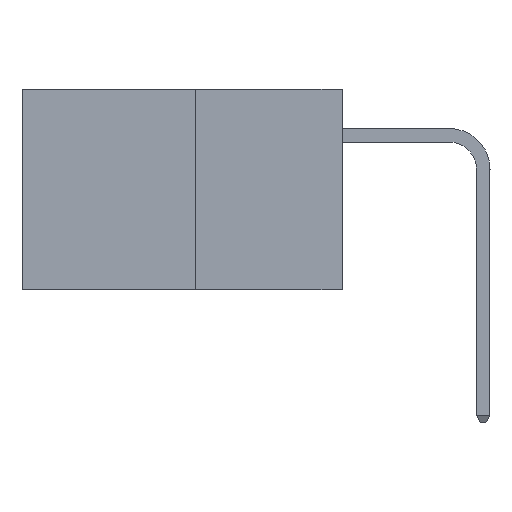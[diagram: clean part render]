
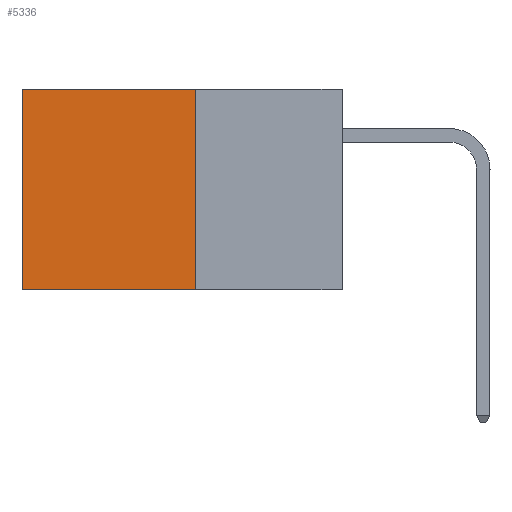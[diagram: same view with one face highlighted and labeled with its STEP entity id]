
A CAD part, left-side view. The second image highlights one B-rep face of the part: STEP entity #5336.
In plain terms, the highlighted planar face has unit normal (-1, 0, 0).
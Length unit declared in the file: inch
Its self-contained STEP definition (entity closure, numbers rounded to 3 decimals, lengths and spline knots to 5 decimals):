
#432 = EDGE_CURVE ( 'NONE', #10959, #10117, #7024, .T. ) ;
#1221 = ORIENTED_EDGE ( 'NONE', *, *, #6345, .F. ) ;
#1594 = ORIENTED_EDGE ( 'NONE', *, *, #6650, .F. ) ;
#2426 = FACE_OUTER_BOUND ( 'NONE', #8781, .T. ) ;
#2506 = CARTESIAN_POINT ( 'NONE',  ( 0.277, 0.27, -0.37 ) ) ;
#2788 = DIRECTION ( 'NONE',  ( 1., 0., 0. ) ) ;
#3275 = DIRECTION ( 'NONE',  ( 0., 0., -1. ) ) ;
#3583 = VECTOR ( 'NONE', #8710, 39.37008 ) ;
#3636 = EDGE_CURVE ( 'NONE', #10117, #7857, #12831, .T. ) ;
#4888 = VECTOR ( 'NONE', #12322, 39.37008 ) ;
#5064 = CARTESIAN_POINT ( 'NONE',  ( 0.277, 0.27, 0. ) ) ;
#5336 = ADVANCED_FACE ( 'NONE', ( #2426 ), #11012, .F. ) ;
#6202 = CARTESIAN_POINT ( 'NONE',  ( 0.277, 0.27, -0.37 ) ) ;
#6314 = LINE ( 'NONE', #2506, #3583 ) ;
#6345 = EDGE_CURVE ( 'NONE', #10959, #6708, #6314, .T. ) ;
#6650 = EDGE_CURVE ( 'NONE', #6708, #7857, #10659, .T. ) ;
#6708 = VERTEX_POINT ( 'NONE', #6202 ) ;
#6890 = CARTESIAN_POINT ( 'NONE',  ( 0.277, 0.59, 0. ) ) ;
#7024 = LINE ( 'NONE', #5064, #12454 ) ;
#7400 = VECTOR ( 'NONE', #3275, 39.37008 ) ;
#7857 = VERTEX_POINT ( 'NONE', #8082 ) ;
#8082 = CARTESIAN_POINT ( 'NONE',  ( 0.277, 0.59, -0.37 ) ) ;
#8710 = DIRECTION ( 'NONE',  ( 0., 0., -1. ) ) ;
#8769 = ORIENTED_EDGE ( 'NONE', *, *, #432, .T. ) ;
#8781 = EDGE_LOOP ( 'NONE', ( #10660, #1594, #1221, #8769 ) ) ;
#8976 = AXIS2_PLACEMENT_3D ( 'NONE', #8977, #2788, #10025 ) ;
#8977 = CARTESIAN_POINT ( 'NONE',  ( 0.277, 0.27, -0.37 ) ) ;
#9412 = CARTESIAN_POINT ( 'NONE',  ( 0.277, 0.59, -0.37 ) ) ;
#10025 = DIRECTION ( 'NONE',  ( 0., 0., -1. ) ) ;
#10117 = VERTEX_POINT ( 'NONE', #6890 ) ;
#10289 = CARTESIAN_POINT ( 'NONE',  ( 0.277, 0.27, 0. ) ) ;
#10300 = CARTESIAN_POINT ( 'NONE',  ( 0.277, 0.27, -0.37 ) ) ;
#10659 = LINE ( 'NONE', #10300, #4888 ) ;
#10660 = ORIENTED_EDGE ( 'NONE', *, *, #3636, .T. ) ;
#10959 = VERTEX_POINT ( 'NONE', #10289 ) ;
#11012 = PLANE ( 'NONE',  #8976 ) ;
#12322 = DIRECTION ( 'NONE',  ( 0., 1., 0. ) ) ;
#12454 = VECTOR ( 'NONE', #12763, 39.37008 ) ;
#12763 = DIRECTION ( 'NONE',  ( 0., 1., 0. ) ) ;
#12831 = LINE ( 'NONE', #9412, #7400 ) ;
